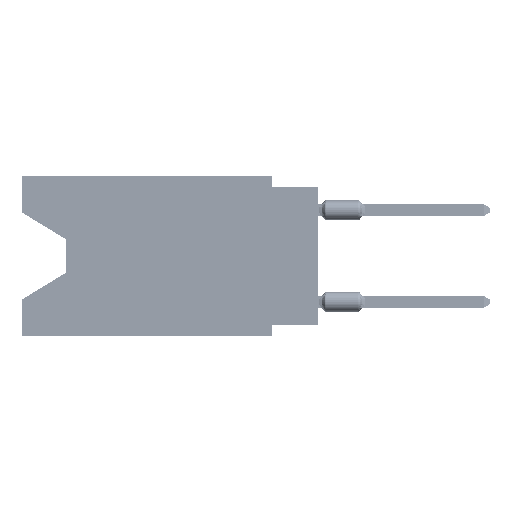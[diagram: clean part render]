
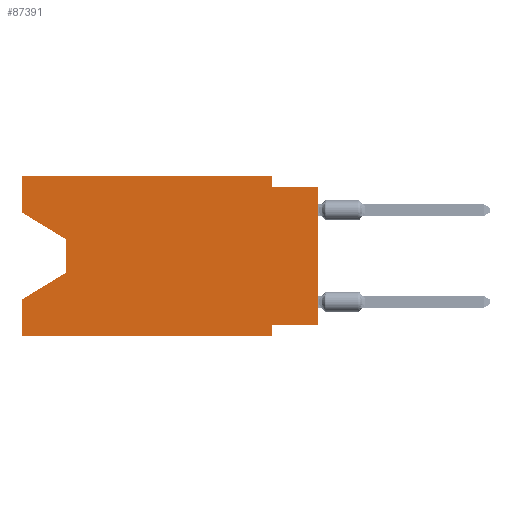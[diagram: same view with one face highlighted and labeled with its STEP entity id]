
A CAD part, left-side view. The second image highlights one B-rep face of the part: STEP entity #87391.
In plain terms, the highlighted planar face has unit normal (-1, 0, 0).
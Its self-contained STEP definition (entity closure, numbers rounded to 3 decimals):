
#754 = CARTESIAN_POINT ( 'NONE',  ( 0., 0., 0. ) ) ;
#2210 = EDGE_CURVE ( 'NONE', #12158, #43139, #23696, .T. ) ;
#2819 = VERTEX_POINT ( 'NONE', #66368 ) ;
#4080 = DIRECTION ( 'NONE',  ( 0., -1., 0. ) ) ;
#4560 = CARTESIAN_POINT ( 'NONE',  ( 0., 0., -8.255 ) ) ;
#4733 = ORIENTED_EDGE ( 'NONE', *, *, #57330, .F. ) ;
#4966 = ORIENTED_EDGE ( 'NONE', *, *, #52244, .F. ) ;
#5125 = EDGE_CURVE ( 'NONE', #29089, #94253, #78053, .T. ) ;
#6965 = VERTEX_POINT ( 'NONE', #64441 ) ;
#7114 = VERTEX_POINT ( 'NONE', #21539 ) ;
#7560 = LINE ( 'NONE', #30993, #13535 ) ;
#7774 = CARTESIAN_POINT ( 'NONE',  ( 0., 16.383, 0. ) ) ;
#9343 = VECTOR ( 'NONE', #13799, 1000. ) ;
#9410 = VECTOR ( 'NONE', #67015, 1000. ) ;
#9746 = CARTESIAN_POINT ( 'NONE',  ( 0., 16.383, -2.038 ) ) ;
#10029 = VECTOR ( 'NONE', #16258, 1000. ) ;
#11946 = EDGE_CURVE ( 'NONE', #12158, #52875, #56920, .T. ) ;
#12158 = VERTEX_POINT ( 'NONE', #86627 ) ;
#13535 = VECTOR ( 'NONE', #37965, 1000. ) ;
#13562 = CARTESIAN_POINT ( 'NONE',  ( 0., 16.383, 0. ) ) ;
#13799 = DIRECTION ( 'NONE',  ( 0., 0., 1. ) ) ;
#16221 = LINE ( 'NONE', #76038, #65712 ) ;
#16258 = DIRECTION ( 'NONE',  ( 0., -0.855, -0.519 ) ) ;
#17431 = LINE ( 'NONE', #25394, #40162 ) ;
#20866 = CARTESIAN_POINT ( 'NONE',  ( 0., 13.97, -3.505 ) ) ;
#21103 = ORIENTED_EDGE ( 'NONE', *, *, #94728, .F. ) ;
#21481 = CARTESIAN_POINT ( 'NONE',  ( 0., 16.383, 0. ) ) ;
#21517 = DIRECTION ( 'NONE',  ( 0., 0.855, -0.519 ) ) ;
#21539 = CARTESIAN_POINT ( 'NONE',  ( 0., 13.97, -5.385 ) ) ;
#22711 = VERTEX_POINT ( 'NONE', #7774 ) ;
#23696 = LINE ( 'NONE', #754, #92382 ) ;
#25394 = CARTESIAN_POINT ( 'NONE',  ( 0., 13.97, -3.505 ) ) ;
#27677 = VECTOR ( 'NONE', #45172, 1000. ) ;
#29089 = VERTEX_POINT ( 'NONE', #55387 ) ;
#30596 = LINE ( 'NONE', #89956, #9410 ) ;
#30993 = CARTESIAN_POINT ( 'NONE',  ( 0., 0., -0.635 ) ) ;
#32212 = VECTOR ( 'NONE', #51871, 1000. ) ;
#32783 = LINE ( 'NONE', #58658, #27677 ) ;
#34570 = VERTEX_POINT ( 'NONE', #69805 ) ;
#35224 = EDGE_CURVE ( 'NONE', #52875, #2819, #32783, .T. ) ;
#35494 = CARTESIAN_POINT ( 'NONE',  ( 0., 13.97, -5.385 ) ) ;
#36460 = LINE ( 'NONE', #35494, #49057 ) ;
#37847 = VERTEX_POINT ( 'NONE', #73469 ) ;
#37965 = DIRECTION ( 'NONE',  ( 0., -1., 0. ) ) ;
#40162 = VECTOR ( 'NONE', #78748, 1000. ) ;
#43139 = VERTEX_POINT ( 'NONE', #90969 ) ;
#45172 = DIRECTION ( 'NONE',  ( 0., 0., -1. ) ) ;
#45914 = DIRECTION ( 'NONE',  ( 0., 0., -1. ) ) ;
#47353 = ORIENTED_EDGE ( 'NONE', *, *, #2210, .T. ) ;
#49057 = VECTOR ( 'NONE', #21517, 1000. ) ;
#49141 = VECTOR ( 'NONE', #65896, 1000. ) ;
#51871 = DIRECTION ( 'NONE',  ( 0., -1., 0. ) ) ;
#51912 = FACE_OUTER_BOUND ( 'NONE', #86054, .T. ) ;
#52244 = EDGE_CURVE ( 'NONE', #34570, #43139, #7560, .T. ) ;
#52875 = VERTEX_POINT ( 'NONE', #57733 ) ;
#53817 = VECTOR ( 'NONE', #4080, 1000. ) ;
#54582 = ORIENTED_EDGE ( 'NONE', *, *, #5125, .T. ) ;
#55387 = CARTESIAN_POINT ( 'NONE',  ( 0., 16.383, -2.038 ) ) ;
#56445 = EDGE_CURVE ( 'NONE', #37847, #2819, #57426, .T. ) ;
#56576 = EDGE_CURVE ( 'NONE', #7114, #6965, #36460, .T. ) ;
#56920 = LINE ( 'NONE', #4560, #49141 ) ;
#57330 = EDGE_CURVE ( 'NONE', #29089, #22711, #97055, .T. ) ;
#57426 = LINE ( 'NONE', #64420, #53817 ) ;
#57733 = CARTESIAN_POINT ( 'NONE',  ( 0., 2.54, -8.255 ) ) ;
#57944 = EDGE_CURVE ( 'NONE', #90978, #34570, #30596, .T. ) ;
#58658 = CARTESIAN_POINT ( 'NONE',  ( 0., 2.54, -8.89 ) ) ;
#59010 = ORIENTED_EDGE ( 'NONE', *, *, #56576, .T. ) ;
#64420 = CARTESIAN_POINT ( 'NONE',  ( 0., 16.383, -8.89 ) ) ;
#64441 = CARTESIAN_POINT ( 'NONE',  ( 0., 16.383, -6.852 ) ) ;
#64874 = ORIENTED_EDGE ( 'NONE', *, *, #35224, .F. ) ;
#65712 = VECTOR ( 'NONE', #84029, 1000. ) ;
#65896 = DIRECTION ( 'NONE',  ( 0., 1., 0. ) ) ;
#66368 = CARTESIAN_POINT ( 'NONE',  ( 0., 2.54, -8.89 ) ) ;
#67015 = DIRECTION ( 'NONE',  ( 0., 0., -1. ) ) ;
#67390 = EDGE_CURVE ( 'NONE', #22711, #90978, #89784, .T. ) ;
#69215 = ORIENTED_EDGE ( 'NONE', *, *, #11946, .F. ) ;
#69551 = DIRECTION ( 'NONE',  ( 0., 0., 1. ) ) ;
#69805 = CARTESIAN_POINT ( 'NONE',  ( 0., 2.54, -0.635 ) ) ;
#73469 = CARTESIAN_POINT ( 'NONE',  ( 0., 16.383, -8.89 ) ) ;
#74869 = ORIENTED_EDGE ( 'NONE', *, *, #67390, .F. ) ;
#75732 = ORIENTED_EDGE ( 'NONE', *, *, #56445, .T. ) ;
#75828 = PLANE ( 'NONE',  #87935 ) ;
#76038 = CARTESIAN_POINT ( 'NONE',  ( 0., 16.383, 0. ) ) ;
#78053 = LINE ( 'NONE', #9746, #10029 ) ;
#78748 = DIRECTION ( 'NONE',  ( 0., 0., -1. ) ) ;
#82023 = ORIENTED_EDGE ( 'NONE', *, *, #57944, .F. ) ;
#82107 = CARTESIAN_POINT ( 'NONE',  ( 0., 16.383, 0. ) ) ;
#82348 = DIRECTION ( 'NONE',  ( 1., 0., 0. ) ) ;
#84029 = DIRECTION ( 'NONE',  ( 0., 0., 1. ) ) ;
#86054 = EDGE_LOOP ( 'NONE', ( #54582, #87581, #59010, #21103, #75732, #64874, #69215, #47353, #4966, #82023, #74869, #4733 ) ) ;
#86627 = CARTESIAN_POINT ( 'NONE',  ( 0., 0., -8.255 ) ) ;
#87391 = ADVANCED_FACE ( 'NONE', ( #51912 ), #75828, .F. ) ;
#87581 = ORIENTED_EDGE ( 'NONE', *, *, #94044, .T. ) ;
#87935 = AXIS2_PLACEMENT_3D ( 'NONE', #13562, #82348, #45914 ) ;
#89130 = CARTESIAN_POINT ( 'NONE',  ( 0., 2.54, 0. ) ) ;
#89784 = LINE ( 'NONE', #21481, #32212 ) ;
#89956 = CARTESIAN_POINT ( 'NONE',  ( 0., 2.54, 0. ) ) ;
#90969 = CARTESIAN_POINT ( 'NONE',  ( 0., 0., -0.635 ) ) ;
#90978 = VERTEX_POINT ( 'NONE', #89130 ) ;
#92382 = VECTOR ( 'NONE', #69551, 1000. ) ;
#94044 = EDGE_CURVE ( 'NONE', #94253, #7114, #17431, .T. ) ;
#94253 = VERTEX_POINT ( 'NONE', #20866 ) ;
#94728 = EDGE_CURVE ( 'NONE', #37847, #6965, #16221, .T. ) ;
#97055 = LINE ( 'NONE', #82107, #9343 ) ;
